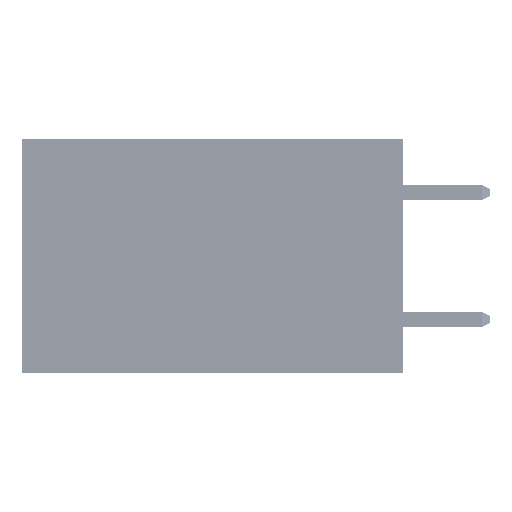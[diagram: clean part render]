
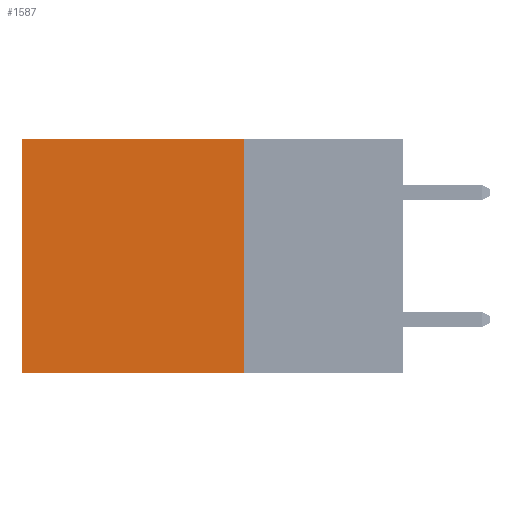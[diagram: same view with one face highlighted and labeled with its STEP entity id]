
A CAD part, left-side view. The second image highlights one B-rep face of the part: STEP entity #1587.
In plain terms, the highlighted planar face has unit normal (-1, 0, 0).
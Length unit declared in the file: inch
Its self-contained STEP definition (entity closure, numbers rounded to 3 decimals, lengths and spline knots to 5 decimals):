
#1587 = ADVANCED_FACE ( 'NONE', ( #25872 ), #41028, .F. ) ;
#1899 = ORIENTED_EDGE ( 'NONE', *, *, #29917, .T. ) ;
#2661 = VECTOR ( 'NONE', #24993, 39.37008 ) ;
#3121 = LINE ( 'NONE', #40862, #5097 ) ;
#5097 = VECTOR ( 'NONE', #18282, 39.37008 ) ;
#7017 = DIRECTION ( 'NONE',  ( 1., 0., 0. ) ) ;
#9858 = CARTESIAN_POINT ( 'NONE',  ( 0.2875, 0.25, 0. ) ) ;
#11235 = DIRECTION ( 'NONE',  ( 0., 0., -1. ) ) ;
#11526 = ORIENTED_EDGE ( 'NONE', *, *, #13862, .F. ) ;
#13862 = EDGE_CURVE ( 'NONE', #15729, #37404, #25728, .T. ) ;
#15729 = VERTEX_POINT ( 'NONE', #30896 ) ;
#16238 = DIRECTION ( 'NONE',  ( 0., 1., 0. ) ) ;
#18282 = DIRECTION ( 'NONE',  ( 0., 1., 0. ) ) ;
#22211 = DIRECTION ( 'NONE',  ( 0., 0., -1. ) ) ;
#23154 = CARTESIAN_POINT ( 'NONE',  ( 0.2875, 0.6, 0. ) ) ;
#23992 = EDGE_CURVE ( 'NONE', #37404, #37591, #38844, .T. ) ;
#24993 = DIRECTION ( 'NONE',  ( 0., 0., -1. ) ) ;
#25465 = CARTESIAN_POINT ( 'NONE',  ( 0.2875, 0.6, 0. ) ) ;
#25728 = LINE ( 'NONE', #9858, #2661 ) ;
#25744 = CARTESIAN_POINT ( 'NONE',  ( 0.2875, 0.25, -0.37 ) ) ;
#25872 = FACE_OUTER_BOUND ( 'NONE', #26842, .T. ) ;
#26842 = EDGE_LOOP ( 'NONE', ( #31209, #34068, #11526, #1899 ) ) ;
#29917 = EDGE_CURVE ( 'NONE', #15729, #30370, #3121, .T. ) ;
#30086 = CARTESIAN_POINT ( 'NONE',  ( 0.2875, 0.25, 0. ) ) ;
#30370 = VERTEX_POINT ( 'NONE', #23154 ) ;
#30896 = CARTESIAN_POINT ( 'NONE',  ( 0.2875, 0.25, 0. ) ) ;
#31209 = ORIENTED_EDGE ( 'NONE', *, *, #40424, .T. ) ;
#34068 = ORIENTED_EDGE ( 'NONE', *, *, #23992, .F. ) ;
#35099 = CARTESIAN_POINT ( 'NONE',  ( 0.2875, 0.25, -0.37 ) ) ;
#37404 = VERTEX_POINT ( 'NONE', #25744 ) ;
#37591 = VERTEX_POINT ( 'NONE', #41031 ) ;
#38787 = VECTOR ( 'NONE', #16238, 39.37008 ) ;
#38844 = LINE ( 'NONE', #35099, #38787 ) ;
#40424 = EDGE_CURVE ( 'NONE', #30370, #37591, #44338, .T. ) ;
#40862 = CARTESIAN_POINT ( 'NONE',  ( 0.2875, 0.25, 0. ) ) ;
#41028 = PLANE ( 'NONE',  #41976 ) ;
#41031 = CARTESIAN_POINT ( 'NONE',  ( 0.2875, 0.6, -0.37 ) ) ;
#41976 = AXIS2_PLACEMENT_3D ( 'NONE', #30086, #7017, #11235 ) ;
#43645 = VECTOR ( 'NONE', #22211, 39.37008 ) ;
#44338 = LINE ( 'NONE', #25465, #43645 ) ;
